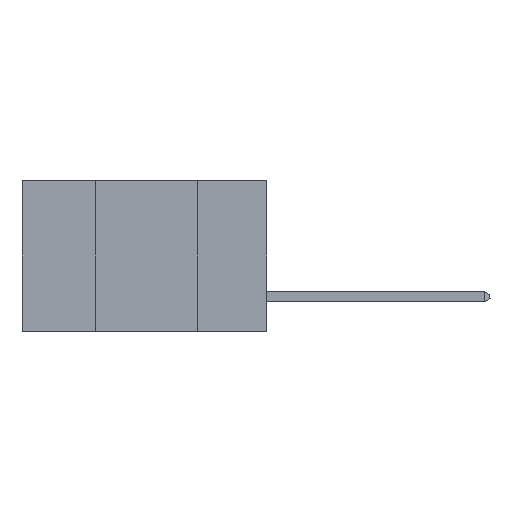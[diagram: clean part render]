
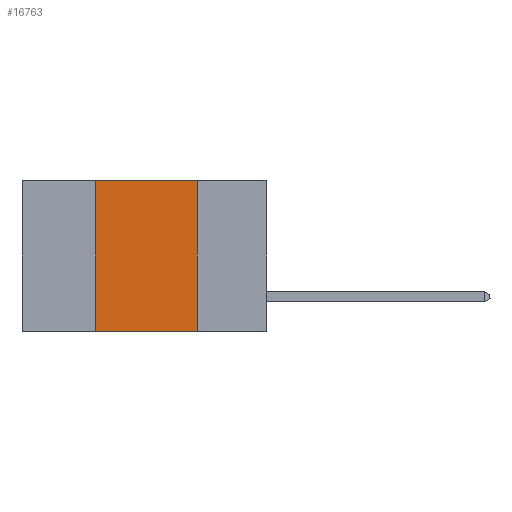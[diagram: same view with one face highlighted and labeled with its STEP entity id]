
A CAD part, left-side view. The second image highlights one B-rep face of the part: STEP entity #16763.
In plain terms, the highlighted planar face has unit normal (-1, 0, 0).
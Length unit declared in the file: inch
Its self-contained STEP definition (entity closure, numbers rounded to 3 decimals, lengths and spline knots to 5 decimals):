
#689 = CARTESIAN_POINT ( 'NONE',  ( 0., 0.17, 0. ) ) ;
#2632 = ORIENTED_EDGE ( 'NONE', *, *, #16924, .F. ) ;
#3393 = VECTOR ( 'NONE', #21121, 39.37008 ) ;
#3668 = VERTEX_POINT ( 'NONE', #13810 ) ;
#4865 = LINE ( 'NONE', #13809, #11720 ) ;
#5241 = DIRECTION ( 'NONE',  ( 0., 0., -1. ) ) ;
#5743 = CARTESIAN_POINT ( 'NONE',  ( 0., 0.6, 0. ) ) ;
#6646 = CARTESIAN_POINT ( 'NONE',  ( 0., 0.17, -0.37 ) ) ;
#8556 = PLANE ( 'NONE',  #16685 ) ;
#11262 = VECTOR ( 'NONE', #17350, 39.37008 ) ;
#11273 = ORIENTED_EDGE ( 'NONE', *, *, #34288, .F. ) ;
#11720 = VECTOR ( 'NONE', #36771, 39.37008 ) ;
#12098 = EDGE_CURVE ( 'NONE', #31939, #34336, #4865, .T. ) ;
#13809 = CARTESIAN_POINT ( 'NONE',  ( 0., 0.6, -0.37 ) ) ;
#13810 = CARTESIAN_POINT ( 'NONE',  ( 0., 0.42, 0. ) ) ;
#15321 = VERTEX_POINT ( 'NONE', #29402 ) ;
#16685 = AXIS2_PLACEMENT_3D ( 'NONE', #5743, #28615, #5241 ) ;
#16763 = ADVANCED_FACE ( 'NONE', ( #18313 ), #8556, .F. ) ;
#16924 = EDGE_CURVE ( 'NONE', #15321, #34336, #36751, .T. ) ;
#17350 = DIRECTION ( 'NONE',  ( 0., -1., 0. ) ) ;
#18120 = ORIENTED_EDGE ( 'NONE', *, *, #12098, .T. ) ;
#18304 = CARTESIAN_POINT ( 'NONE',  ( 0., 0.42, 0. ) ) ;
#18313 = FACE_OUTER_BOUND ( 'NONE', #28558, .T. ) ;
#20091 = CARTESIAN_POINT ( 'NONE',  ( 0., 0.42, -0.37 ) ) ;
#21121 = DIRECTION ( 'NONE',  ( 0., 0., -1. ) ) ;
#21837 = VECTOR ( 'NONE', #30143, 39.37008 ) ;
#24403 = ORIENTED_EDGE ( 'NONE', *, *, #37500, .F. ) ;
#28558 = EDGE_LOOP ( 'NONE', ( #2632, #24403, #11273, #18120 ) ) ;
#28615 = DIRECTION ( 'NONE',  ( 1., 0., 0. ) ) ;
#29402 = CARTESIAN_POINT ( 'NONE',  ( 0., 0.17, 0. ) ) ;
#30042 = LINE ( 'NONE', #18304, #21837 ) ;
#30143 = DIRECTION ( 'NONE',  ( 0., 0., 1. ) ) ;
#31752 = CARTESIAN_POINT ( 'NONE',  ( 0., 0.6, 0. ) ) ;
#31939 = VERTEX_POINT ( 'NONE', #20091 ) ;
#32269 = LINE ( 'NONE', #31752, #11262 ) ;
#34288 = EDGE_CURVE ( 'NONE', #31939, #3668, #30042, .T. ) ;
#34336 = VERTEX_POINT ( 'NONE', #6646 ) ;
#36751 = LINE ( 'NONE', #689, #3393 ) ;
#36771 = DIRECTION ( 'NONE',  ( 0., -1., 0. ) ) ;
#37500 = EDGE_CURVE ( 'NONE', #3668, #15321, #32269, .T. ) ;
